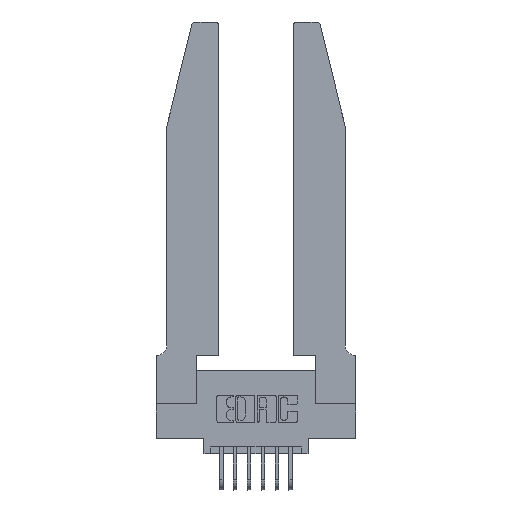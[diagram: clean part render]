
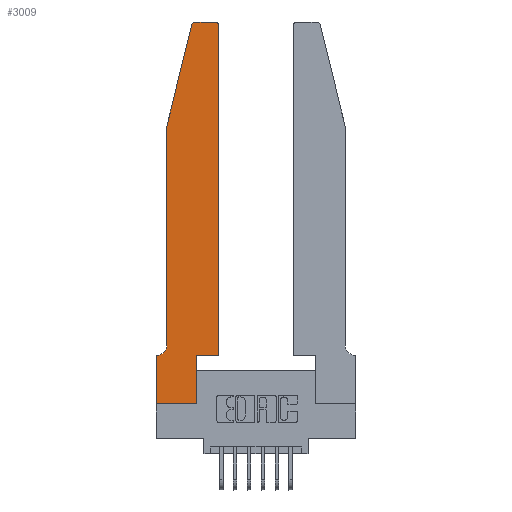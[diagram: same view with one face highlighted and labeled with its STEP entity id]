
A CAD part, top view. The second image highlights one B-rep face of the part: STEP entity #3009.
In plain terms, the highlighted planar face has unit normal (0, 0, 1).
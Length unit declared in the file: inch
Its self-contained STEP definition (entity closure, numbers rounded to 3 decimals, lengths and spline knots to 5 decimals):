
#124 = CARTESIAN_POINT ( 'NONE',  ( 0.2865, 0., 0.37 ) ) ;
#210 = VECTOR ( 'NONE', #9268, 39.37008 ) ;
#751 = ORIENTED_EDGE ( 'NONE', *, *, #4705, .T. ) ;
#927 = CARTESIAN_POINT ( 'NONE',  ( 0., 0.35, 0.37 ) ) ;
#939 = ORIENTED_EDGE ( 'NONE', *, *, #2430, .T. ) ;
#940 = EDGE_CURVE ( 'NONE', #6750, #13396, #3550, .T. ) ;
#1351 = CARTESIAN_POINT ( 'NONE',  ( 0.284, 2.72, 0.37 ) ) ;
#1367 = ORIENTED_EDGE ( 'NONE', *, *, #940, .T. ) ;
#1396 = FACE_OUTER_BOUND ( 'NONE', #4469, .T. ) ;
#1740 = VERTEX_POINT ( 'NONE', #5881 ) ;
#1872 = VERTEX_POINT ( 'NONE', #4133 ) ;
#2367 = AXIS2_PLACEMENT_3D ( 'NONE', #927, #11750, #11597 ) ;
#2430 = EDGE_CURVE ( 'NONE', #3225, #14099, #3314, .T. ) ;
#2589 = DIRECTION ( 'NONE',  ( 1., 0., 0. ) ) ;
#3009 = ADVANCED_FACE ( 'NONE', ( #1396 ), #11121, .T. ) ;
#3215 = CARTESIAN_POINT ( 'NONE',  ( 0.2865, 0.35, 0.37 ) ) ;
#3225 = VERTEX_POINT ( 'NONE', #7360 ) ;
#3314 = LINE ( 'NONE', #10861, #6298 ) ;
#3489 = EDGE_CURVE ( 'NONE', #15767, #9441, #8828, .T. ) ;
#3550 = LINE ( 'NONE', #8344, #210 ) ;
#3665 = CARTESIAN_POINT ( 'NONE',  ( 0.2865, 0.35, 0.37 ) ) ;
#3704 = CARTESIAN_POINT ( 'NONE',  ( 0.4505, 0.35, 0.37 ) ) ;
#3728 = EDGE_CURVE ( 'NONE', #1872, #3225, #8207, .T. ) ;
#4133 = CARTESIAN_POINT ( 'NONE',  ( 0.4505, 2.72, 0.37 ) ) ;
#4334 = CARTESIAN_POINT ( 'NONE',  ( 0.0755, 2., 0.37 ) ) ;
#4469 = EDGE_LOOP ( 'NONE', ( #939, #9605, #8530, #10991, #751, #9295, #1367, #4802, #7940, #5289, #10307, #9964 ) ) ;
#4585 = VECTOR ( 'NONE', #5721, 39.37008 ) ;
#4705 = EDGE_CURVE ( 'NONE', #9441, #1740, #5627, .T. ) ;
#4802 = ORIENTED_EDGE ( 'NONE', *, *, #11395, .T. ) ;
#4890 = EDGE_CURVE ( 'NONE', #11139, #1872, #13207, .T. ) ;
#4893 = CARTESIAN_POINT ( 'NONE',  ( 0., 0.35, 0.37 ) ) ;
#5211 = VECTOR ( 'NONE', #10703, 39.37008 ) ;
#5242 = EDGE_CURVE ( 'NONE', #14099, #7596, #8564, .T. ) ;
#5289 = ORIENTED_EDGE ( 'NONE', *, *, #12570, .T. ) ;
#5329 = VECTOR ( 'NONE', #7909, 39.37008 ) ;
#5371 = CARTESIAN_POINT ( 'NONE',  ( 0.0755, 0.35, 0.37 ) ) ;
#5483 = CARTESIAN_POINT ( 'NONE',  ( 0.4205, 2.72, 0.37 ) ) ;
#5627 = CIRCLE ( 'NONE', #14122, 0.07 ) ;
#5721 = DIRECTION ( 'NONE',  ( -0.239, -0.971, 0. ) ) ;
#5881 = CARTESIAN_POINT ( 'NONE',  ( 0.0055, 0.35, 0.37 ) ) ;
#5963 = VECTOR ( 'NONE', #12817, 39.37008 ) ;
#6007 = CARTESIAN_POINT ( 'NONE',  ( 0.0055, 0.42, 0.37 ) ) ;
#6298 = VECTOR ( 'NONE', #10386, 39.37008 ) ;
#6608 = EDGE_CURVE ( 'NONE', #11851, #13659, #14702, .T. ) ;
#6741 = DIRECTION ( 'NONE',  ( 1., 0., 0. ) ) ;
#6750 = VERTEX_POINT ( 'NONE', #4893 ) ;
#7247 = VECTOR ( 'NONE', #11602, 39.37008 ) ;
#7272 = DIRECTION ( 'NONE',  ( -1., 0., 0. ) ) ;
#7360 = CARTESIAN_POINT ( 'NONE',  ( 0.4205, 2.75, 0.37 ) ) ;
#7596 = VERTEX_POINT ( 'NONE', #12805 ) ;
#7909 = DIRECTION ( 'NONE',  ( 1., 0., 0. ) ) ;
#7940 = ORIENTED_EDGE ( 'NONE', *, *, #6608, .T. ) ;
#8087 = CARTESIAN_POINT ( 'NONE',  ( 0., 0., 0.37 ) ) ;
#8207 = CIRCLE ( 'NONE', #13414, 0.03 ) ;
#8344 = CARTESIAN_POINT ( 'NONE',  ( 0., 0., 0.37 ) ) ;
#8374 = EDGE_CURVE ( 'NONE', #7596, #15767, #14842, .T. ) ;
#8530 = ORIENTED_EDGE ( 'NONE', *, *, #8374, .T. ) ;
#8564 = CIRCLE ( 'NONE', #10240, 0.03 ) ;
#8651 = CARTESIAN_POINT ( 'NONE',  ( 0.0755, 0.42, 0.37 ) ) ;
#8828 = LINE ( 'NONE', #4334, #7247 ) ;
#8918 = CARTESIAN_POINT ( 'NONE',  ( 0.4505, 0.35, 0.37 ) ) ;
#9146 = CARTESIAN_POINT ( 'NONE',  ( 0., 0., 0.37 ) ) ;
#9268 = DIRECTION ( 'NONE',  ( 0., -1., 0. ) ) ;
#9295 = ORIENTED_EDGE ( 'NONE', *, *, #10172, .T. ) ;
#9441 = VERTEX_POINT ( 'NONE', #8651 ) ;
#9605 = ORIENTED_EDGE ( 'NONE', *, *, #5242, .T. ) ;
#9964 = ORIENTED_EDGE ( 'NONE', *, *, #3728, .T. ) ;
#10107 = DIRECTION ( 'NONE',  ( 0., 0., 1. ) ) ;
#10172 = EDGE_CURVE ( 'NONE', #1740, #6750, #12952, .T. ) ;
#10240 = AXIS2_PLACEMENT_3D ( 'NONE', #1351, #10107, #2589 ) ;
#10307 = ORIENTED_EDGE ( 'NONE', *, *, #4890, .T. ) ;
#10386 = DIRECTION ( 'NONE',  ( -1., 0., 0. ) ) ;
#10703 = DIRECTION ( 'NONE',  ( 0., 1., 0. ) ) ;
#10861 = CARTESIAN_POINT ( 'NONE',  ( 0.2605, 2.75, 0.37 ) ) ;
#10991 = ORIENTED_EDGE ( 'NONE', *, *, #3489, .T. ) ;
#11121 = PLANE ( 'NONE',  #2367 ) ;
#11139 = VERTEX_POINT ( 'NONE', #14871 ) ;
#11395 = EDGE_CURVE ( 'NONE', #13396, #11851, #11950, .T. ) ;
#11597 = DIRECTION ( 'NONE',  ( 1., 0., 0. ) ) ;
#11602 = DIRECTION ( 'NONE',  ( 0., -1., 0. ) ) ;
#11750 = DIRECTION ( 'NONE',  ( 0., 0., 1. ) ) ;
#11851 = VERTEX_POINT ( 'NONE', #124 ) ;
#11940 = LINE ( 'NONE', #3704, #15175 ) ;
#11950 = LINE ( 'NONE', #9146, #5329 ) ;
#11988 = CARTESIAN_POINT ( 'NONE',  ( 0.0755, 2., 0.37 ) ) ;
#12453 = DIRECTION ( 'NONE',  ( 1., 0., 0. ) ) ;
#12570 = EDGE_CURVE ( 'NONE', #13659, #11139, #11940, .T. ) ;
#12805 = CARTESIAN_POINT ( 'NONE',  ( 0.25487, 2.72718, 0.37 ) ) ;
#12817 = DIRECTION ( 'NONE',  ( -1., 0., 0. ) ) ;
#12952 = LINE ( 'NONE', #5371, #5963 ) ;
#13207 = LINE ( 'NONE', #8918, #16041 ) ;
#13396 = VERTEX_POINT ( 'NONE', #8087 ) ;
#13414 = AXIS2_PLACEMENT_3D ( 'NONE', #5483, #14138, #6741 ) ;
#13659 = VERTEX_POINT ( 'NONE', #3665 ) ;
#14099 = VERTEX_POINT ( 'NONE', #15845 ) ;
#14122 = AXIS2_PLACEMENT_3D ( 'NONE', #6007, #14651, #7272 ) ;
#14138 = DIRECTION ( 'NONE',  ( 0., 0., 1. ) ) ;
#14379 = CARTESIAN_POINT ( 'NONE',  ( 0.0755, 2., 0.37 ) ) ;
#14651 = DIRECTION ( 'NONE',  ( 0., 0., -1. ) ) ;
#14702 = LINE ( 'NONE', #3215, #5211 ) ;
#14842 = LINE ( 'NONE', #14379, #4585 ) ;
#14871 = CARTESIAN_POINT ( 'NONE',  ( 0.4505, 0.35, 0.37 ) ) ;
#15028 = DIRECTION ( 'NONE',  ( 0., 1., 0. ) ) ;
#15175 = VECTOR ( 'NONE', #12453, 39.37008 ) ;
#15767 = VERTEX_POINT ( 'NONE', #11988 ) ;
#15845 = CARTESIAN_POINT ( 'NONE',  ( 0.284, 2.75, 0.37 ) ) ;
#16041 = VECTOR ( 'NONE', #15028, 39.37008 ) ;
